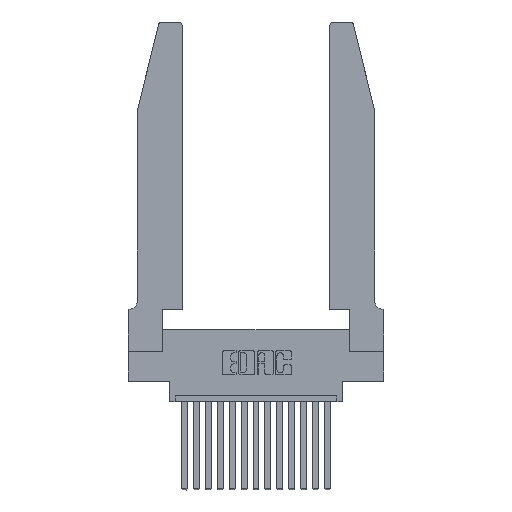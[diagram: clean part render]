
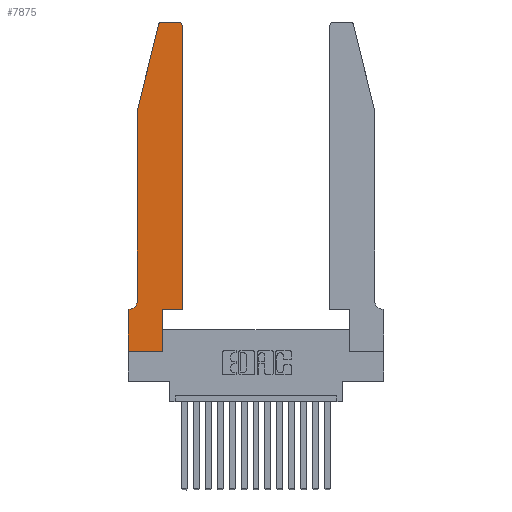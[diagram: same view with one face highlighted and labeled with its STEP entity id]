
A CAD part, top view. The second image highlights one B-rep face of the part: STEP entity #7875.
In plain terms, the highlighted planar face has unit normal (0, 0, 1).
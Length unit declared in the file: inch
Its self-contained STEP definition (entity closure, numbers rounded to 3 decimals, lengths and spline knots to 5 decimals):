
#169 = LINE ( 'NONE', #2036, #13498 ) ;
#320 = CIRCLE ( 'NONE', #8711, 0.07 ) ;
#435 = ORIENTED_EDGE ( 'NONE', *, *, #11360, .T. ) ;
#495 = DIRECTION ( 'NONE',  ( 1., 0., 0. ) ) ;
#712 = CARTESIAN_POINT ( 'NONE',  ( 0.0755, 0.42, 0.37 ) ) ;
#1394 = ORIENTED_EDGE ( 'NONE', *, *, #10695, .T. ) ;
#1447 = CARTESIAN_POINT ( 'NONE',  ( 0.0055, 0.35, 0.37 ) ) ;
#1512 = AXIS2_PLACEMENT_3D ( 'NONE', #9759, #5405, #15299 ) ;
#1552 = DIRECTION ( 'NONE',  ( 1., 0., 0. ) ) ;
#1701 = LINE ( 'NONE', #16699, #2167 ) ;
#1782 = EDGE_CURVE ( 'NONE', #4959, #3410, #320, .T. ) ;
#1833 = CIRCLE ( 'NONE', #8078, 0.03 ) ;
#2036 = CARTESIAN_POINT ( 'NONE',  ( 0.0755, 2., 0.37 ) ) ;
#2167 = VECTOR ( 'NONE', #11125, 39.37008 ) ;
#2771 = LINE ( 'NONE', #15017, #17662 ) ;
#3279 = VERTEX_POINT ( 'NONE', #17205 ) ;
#3333 = ORIENTED_EDGE ( 'NONE', *, *, #4424, .T. ) ;
#3390 = CARTESIAN_POINT ( 'NONE',  ( 0.4505, 2.72, 0.37 ) ) ;
#3410 = VERTEX_POINT ( 'NONE', #1447 ) ;
#3707 = ORIENTED_EDGE ( 'NONE', *, *, #14165, .T. ) ;
#4172 = LINE ( 'NONE', #13656, #8839 ) ;
#4424 = EDGE_CURVE ( 'NONE', #5441, #7389, #4172, .T. ) ;
#4479 = CARTESIAN_POINT ( 'NONE',  ( 0., 0., 0.37 ) ) ;
#4493 = VERTEX_POINT ( 'NONE', #10946 ) ;
#4768 = EDGE_CURVE ( 'NONE', #3410, #11950, #11705, .T. ) ;
#4959 = VERTEX_POINT ( 'NONE', #712 ) ;
#5405 = DIRECTION ( 'NONE',  ( 0., 0., 1. ) ) ;
#5438 = VERTEX_POINT ( 'NONE', #5740 ) ;
#5441 = VERTEX_POINT ( 'NONE', #17099 ) ;
#5740 = CARTESIAN_POINT ( 'NONE',  ( 0.4205, 2.75, 0.37 ) ) ;
#5752 = VECTOR ( 'NONE', #8648, 39.37008 ) ;
#6118 = ORIENTED_EDGE ( 'NONE', *, *, #16193, .T. ) ;
#6317 = DIRECTION ( 'NONE',  ( 0., -1., 0. ) ) ;
#6763 = DIRECTION ( 'NONE',  ( 0., 0., -1. ) ) ;
#6900 = DIRECTION ( 'NONE',  ( 0., 1., 0. ) ) ;
#7025 = CARTESIAN_POINT ( 'NONE',  ( 0.4505, 0.35, 0.37 ) ) ;
#7079 = EDGE_CURVE ( 'NONE', #7461, #16081, #16940, .T. ) ;
#7389 = VERTEX_POINT ( 'NONE', #8044 ) ;
#7461 = VERTEX_POINT ( 'NONE', #15372 ) ;
#7608 = CARTESIAN_POINT ( 'NONE',  ( 0., 0.35, 0.37 ) ) ;
#7667 = CARTESIAN_POINT ( 'NONE',  ( 0., 0., 0.37 ) ) ;
#7849 = CIRCLE ( 'NONE', #18221, 0.03 ) ;
#7875 = ADVANCED_FACE ( 'NONE', ( #8263 ), #13867, .T. ) ;
#8044 = CARTESIAN_POINT ( 'NONE',  ( 0.0755, 2., 0.37 ) ) ;
#8078 = AXIS2_PLACEMENT_3D ( 'NONE', #14256, #10090, #1552 ) ;
#8090 = CARTESIAN_POINT ( 'NONE',  ( 0.284, 2.72, 0.37 ) ) ;
#8263 = FACE_OUTER_BOUND ( 'NONE', #14446, .T. ) ;
#8648 = DIRECTION ( 'NONE',  ( 0., 1., 0. ) ) ;
#8669 = ORIENTED_EDGE ( 'NONE', *, *, #1782, .T. ) ;
#8711 = AXIS2_PLACEMENT_3D ( 'NONE', #13735, #6763, #17980 ) ;
#8819 = VERTEX_POINT ( 'NONE', #4479 ) ;
#8839 = VECTOR ( 'NONE', #16529, 39.37008 ) ;
#9064 = CARTESIAN_POINT ( 'NONE',  ( 0.0755, 0.35, 0.37 ) ) ;
#9328 = DIRECTION ( 'NONE',  ( 1., 0., 0. ) ) ;
#9519 = LINE ( 'NONE', #14172, #5752 ) ;
#9614 = DIRECTION ( 'NONE',  ( 0., 0., 1. ) ) ;
#9759 = CARTESIAN_POINT ( 'NONE',  ( 0., 0.35, 0.37 ) ) ;
#9951 = ORIENTED_EDGE ( 'NONE', *, *, #16835, .T. ) ;
#10090 = DIRECTION ( 'NONE',  ( 0., 0., 1. ) ) ;
#10695 = EDGE_CURVE ( 'NONE', #5438, #17332, #1701, .T. ) ;
#10946 = CARTESIAN_POINT ( 'NONE',  ( 0.2865, 0.35, 0.37 ) ) ;
#11125 = DIRECTION ( 'NONE',  ( -1., 0., 0. ) ) ;
#11360 = EDGE_CURVE ( 'NONE', #17332, #5441, #7849, .T. ) ;
#11495 = VECTOR ( 'NONE', #15925, 39.37008 ) ;
#11705 = LINE ( 'NONE', #9064, #11495 ) ;
#11950 = VERTEX_POINT ( 'NONE', #7608 ) ;
#12111 = CARTESIAN_POINT ( 'NONE',  ( 0.284, 2.75, 0.37 ) ) ;
#12299 = ORIENTED_EDGE ( 'NONE', *, *, #7079, .T. ) ;
#12301 = EDGE_CURVE ( 'NONE', #8819, #3279, #17552, .T. ) ;
#13498 = VECTOR ( 'NONE', #15037, 39.37008 ) ;
#13632 = CARTESIAN_POINT ( 'NONE',  ( 0.4505, 0.35, 0.37 ) ) ;
#13656 = CARTESIAN_POINT ( 'NONE',  ( 0.0755, 2., 0.37 ) ) ;
#13735 = CARTESIAN_POINT ( 'NONE',  ( 0.0055, 0.42, 0.37 ) ) ;
#13854 = DIRECTION ( 'NONE',  ( 1., 0., 0. ) ) ;
#13867 = PLANE ( 'NONE',  #1512 ) ;
#14090 = EDGE_CURVE ( 'NONE', #7389, #4959, #169, .T. ) ;
#14165 = EDGE_CURVE ( 'NONE', #4493, #7461, #17711, .T. ) ;
#14172 = CARTESIAN_POINT ( 'NONE',  ( 0.2865, 0.35, 0.37 ) ) ;
#14245 = EDGE_CURVE ( 'NONE', #3279, #4493, #9519, .T. ) ;
#14256 = CARTESIAN_POINT ( 'NONE',  ( 0.4205, 2.72, 0.37 ) ) ;
#14277 = ORIENTED_EDGE ( 'NONE', *, *, #14245, .T. ) ;
#14446 = EDGE_LOOP ( 'NONE', ( #1394, #435, #3333, #17902, #8669, #17064, #6118, #14985, #14277, #3707, #12299, #9951 ) ) ;
#14985 = ORIENTED_EDGE ( 'NONE', *, *, #12301, .T. ) ;
#15017 = CARTESIAN_POINT ( 'NONE',  ( 0., 0., 0.37 ) ) ;
#15037 = DIRECTION ( 'NONE',  ( 0., -1., 0. ) ) ;
#15299 = DIRECTION ( 'NONE',  ( 1., 0., 0. ) ) ;
#15372 = CARTESIAN_POINT ( 'NONE',  ( 0.4505, 0.35, 0.37 ) ) ;
#15925 = DIRECTION ( 'NONE',  ( -1., 0., 0. ) ) ;
#16081 = VERTEX_POINT ( 'NONE', #3390 ) ;
#16193 = EDGE_CURVE ( 'NONE', #11950, #8819, #2771, .T. ) ;
#16195 = VECTOR ( 'NONE', #495, 39.37008 ) ;
#16480 = VECTOR ( 'NONE', #6900, 39.37008 ) ;
#16529 = DIRECTION ( 'NONE',  ( -0.239, -0.971, 0. ) ) ;
#16699 = CARTESIAN_POINT ( 'NONE',  ( 0.2605, 2.75, 0.37 ) ) ;
#16835 = EDGE_CURVE ( 'NONE', #16081, #5438, #1833, .T. ) ;
#16940 = LINE ( 'NONE', #7025, #16480 ) ;
#17064 = ORIENTED_EDGE ( 'NONE', *, *, #4768, .T. ) ;
#17099 = CARTESIAN_POINT ( 'NONE',  ( 0.25487, 2.72718, 0.37 ) ) ;
#17205 = CARTESIAN_POINT ( 'NONE',  ( 0.2865, 0., 0.37 ) ) ;
#17332 = VERTEX_POINT ( 'NONE', #12111 ) ;
#17523 = VECTOR ( 'NONE', #9328, 39.37008 ) ;
#17552 = LINE ( 'NONE', #7667, #16195 ) ;
#17662 = VECTOR ( 'NONE', #6317, 39.37008 ) ;
#17711 = LINE ( 'NONE', #13632, #17523 ) ;
#17902 = ORIENTED_EDGE ( 'NONE', *, *, #14090, .T. ) ;
#17980 = DIRECTION ( 'NONE',  ( -1., 0., 0. ) ) ;
#18221 = AXIS2_PLACEMENT_3D ( 'NONE', #8090, #9614, #13854 ) ;
